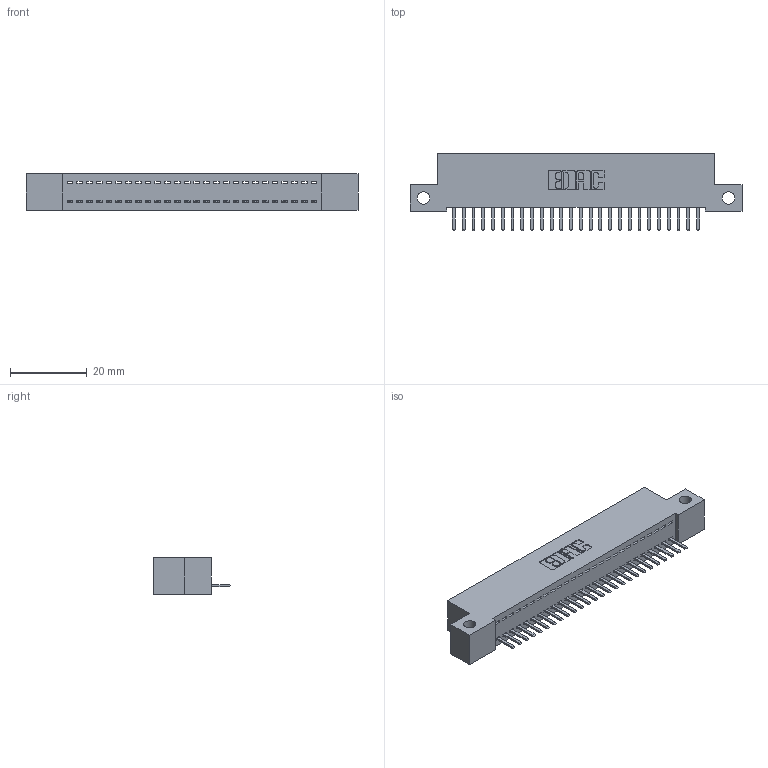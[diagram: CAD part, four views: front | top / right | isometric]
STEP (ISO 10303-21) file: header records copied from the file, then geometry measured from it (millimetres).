
FILE_DESCRIPTION (( 'STEP AP203' ), '1' );
FILE_NAME ('392-026-520-112.STEP', '2018-08-15T15:05:26', ( '' ), ( '' ), 'SwSTEP 2.0', 'SolidWorks 2016', '' );
FILE_SCHEMA (( 'CONFIG_CONTROL_DESIGN' ));
Length unit declared in the file: inch
Products named in the file (3): 342 Part_Side Mount; 345-292-001_345-293-120; 392-026-520-112
Assembly tree (27 placements, depth 2):
  392-026-520-112
    342 Part_Side Mount
    345-292-001_345-293-120  x26
Bounding box: 86.36 x 20.02 x 9.4 mm (x, y, z)
Volume: 7364.4 mm3; surface area: 10113.2 mm2
Topology: 27 solids, 27 shells, 1722 faces, 5083 edges, 3318 vertices
Faces by surface type: plane 1210, cylinder 512
Entity records: 17949 total; most frequent: CARTESIAN_POINT 3116, ORIENTED_EDGE 3066, DIRECTION 2649, EDGE_CURVE 1533, VECTOR 1401, LINE 1401, VERTEX_POINT 1018, AXIS2_PLACEMENT_3D 624
